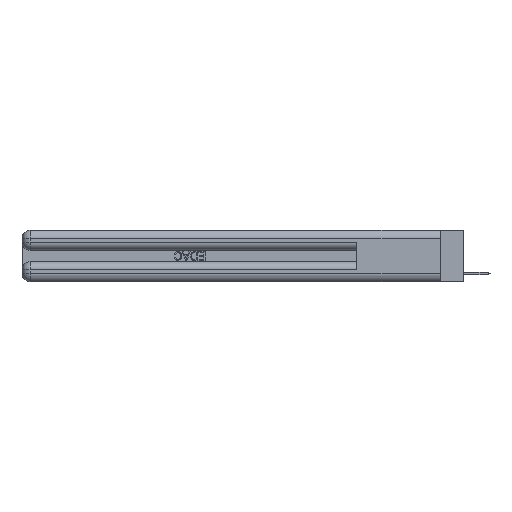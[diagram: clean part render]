
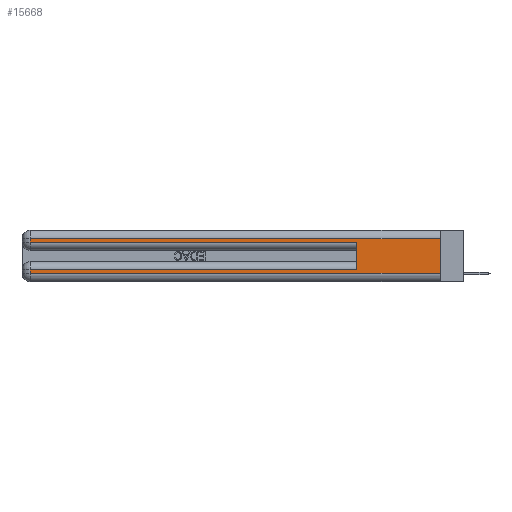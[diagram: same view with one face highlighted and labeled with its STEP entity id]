
A CAD part, left-side view. The second image highlights one B-rep face of the part: STEP entity #15668.
In plain terms, the highlighted planar face has unit normal (-1, 0, 0).
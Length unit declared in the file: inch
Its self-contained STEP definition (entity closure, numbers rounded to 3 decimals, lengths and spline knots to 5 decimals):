
#239 = VECTOR ( 'NONE', #15627, 39.37008 ) ;
#429 = CARTESIAN_POINT ( 'NONE',  ( 0., 0., 0.31 ) ) ;
#573 = EDGE_CURVE ( 'NONE', #22714, #7051, #14240, .T. ) ;
#1526 = ORIENTED_EDGE ( 'NONE', *, *, #16841, .T. ) ;
#1553 = VERTEX_POINT ( 'NONE', #7938 ) ;
#2909 = CARTESIAN_POINT ( 'NONE',  ( 0., 2.94, 0.31 ) ) ;
#2982 = CARTESIAN_POINT ( 'NONE',  ( 0., 0., 0.285 ) ) ;
#3354 = PLANE ( 'NONE',  #17115 ) ;
#3477 = ORIENTED_EDGE ( 'NONE', *, *, #8766, .T. ) ;
#3708 = ORIENTED_EDGE ( 'NONE', *, *, #11903, .T. ) ;
#3887 = EDGE_LOOP ( 'NONE', ( #17079, #9381, #19262, #3708, #11770, #1526, #8779, #3477 ) ) ;
#4520 = VECTOR ( 'NONE', #27031, 39.37008 ) ;
#4703 = CARTESIAN_POINT ( 'NONE',  ( 0., 2.94, 0.285 ) ) ;
#4941 = VERTEX_POINT ( 'NONE', #2909 ) ;
#5452 = CARTESIAN_POINT ( 'NONE',  ( 0., 0.6, 0.145 ) ) ;
#5494 = DIRECTION ( 'NONE',  ( 0., 0., -1. ) ) ;
#5507 = EDGE_CURVE ( 'NONE', #13946, #19288, #10993, .T. ) ;
#6389 = CARTESIAN_POINT ( 'NONE',  ( 0., 0.6, 0.085 ) ) ;
#7051 = VERTEX_POINT ( 'NONE', #27505 ) ;
#7171 = VECTOR ( 'NONE', #9244, 39.37008 ) ;
#7185 = CARTESIAN_POINT ( 'NONE',  ( 0., 2.94, 0.37 ) ) ;
#7938 = CARTESIAN_POINT ( 'NONE',  ( 0., 0.6, 0.285 ) ) ;
#8766 = EDGE_CURVE ( 'NONE', #19288, #7051, #10172, .T. ) ;
#8779 = ORIENTED_EDGE ( 'NONE', *, *, #5507, .T. ) ;
#8797 = LINE ( 'NONE', #5452, #7171 ) ;
#8917 = EDGE_CURVE ( 'NONE', #22714, #4941, #16277, .T. ) ;
#9050 = FACE_OUTER_BOUND ( 'NONE', #3887, .T. ) ;
#9244 = DIRECTION ( 'NONE',  ( 0., 0., 1. ) ) ;
#9381 = ORIENTED_EDGE ( 'NONE', *, *, #8917, .T. ) ;
#9525 = DIRECTION ( 'NONE',  ( 0., 1., 0. ) ) ;
#10096 = DIRECTION ( 'NONE',  ( 0., 0., -1. ) ) ;
#10172 = LINE ( 'NONE', #11922, #4520 ) ;
#10226 = VECTOR ( 'NONE', #11523, 39.37008 ) ;
#10326 = VECTOR ( 'NONE', #19704, 39.37008 ) ;
#10636 = CARTESIAN_POINT ( 'NONE',  ( 0., 0., 0.31 ) ) ;
#10993 = LINE ( 'NONE', #7185, #10326 ) ;
#11523 = DIRECTION ( 'NONE',  ( 0., -1., 0. ) ) ;
#11770 = ORIENTED_EDGE ( 'NONE', *, *, #24814, .F. ) ;
#11775 = CARTESIAN_POINT ( 'NONE',  ( 0., 2.94, 0.37 ) ) ;
#11903 = EDGE_CURVE ( 'NONE', #18441, #1553, #27255, .T. ) ;
#11922 = CARTESIAN_POINT ( 'NONE',  ( 0., 0., 0.06 ) ) ;
#12849 = CARTESIAN_POINT ( 'NONE',  ( 0., 2.94, 0.085 ) ) ;
#13946 = VERTEX_POINT ( 'NONE', #12849 ) ;
#14240 = LINE ( 'NONE', #21968, #239 ) ;
#14255 = CARTESIAN_POINT ( 'NONE',  ( 0., 2.94, 0.06 ) ) ;
#14999 = VECTOR ( 'NONE', #18984, 39.37008 ) ;
#15140 = LINE ( 'NONE', #11775, #25824 ) ;
#15627 = DIRECTION ( 'NONE',  ( 0., 0., -1. ) ) ;
#15668 = ADVANCED_FACE ( 'NONE', ( #9050 ), #3354, .F. ) ;
#16277 = LINE ( 'NONE', #10636, #26973 ) ;
#16841 = EDGE_CURVE ( 'NONE', #20194, #13946, #19969, .T. ) ;
#17079 = ORIENTED_EDGE ( 'NONE', *, *, #573, .F. ) ;
#17115 = AXIS2_PLACEMENT_3D ( 'NONE', #22604, #24765, #5494 ) ;
#18441 = VERTEX_POINT ( 'NONE', #4703 ) ;
#18984 = DIRECTION ( 'NONE',  ( 0., 1., 0. ) ) ;
#19262 = ORIENTED_EDGE ( 'NONE', *, *, #21083, .T. ) ;
#19288 = VERTEX_POINT ( 'NONE', #14255 ) ;
#19704 = DIRECTION ( 'NONE',  ( 0., 0., -1. ) ) ;
#19969 = LINE ( 'NONE', #25441, #14999 ) ;
#20194 = VERTEX_POINT ( 'NONE', #6389 ) ;
#21083 = EDGE_CURVE ( 'NONE', #4941, #18441, #15140, .T. ) ;
#21968 = CARTESIAN_POINT ( 'NONE',  ( 0., 0., 0.37 ) ) ;
#22604 = CARTESIAN_POINT ( 'NONE',  ( 0., 0., 0.37 ) ) ;
#22714 = VERTEX_POINT ( 'NONE', #429 ) ;
#24765 = DIRECTION ( 'NONE',  ( 1., 0., 0. ) ) ;
#24814 = EDGE_CURVE ( 'NONE', #20194, #1553, #8797, .T. ) ;
#25441 = CARTESIAN_POINT ( 'NONE',  ( 0., 0., 0.085 ) ) ;
#25824 = VECTOR ( 'NONE', #10096, 39.37008 ) ;
#26973 = VECTOR ( 'NONE', #9525, 39.37008 ) ;
#27031 = DIRECTION ( 'NONE',  ( 0., -1., 0. ) ) ;
#27255 = LINE ( 'NONE', #2982, #10226 ) ;
#27505 = CARTESIAN_POINT ( 'NONE',  ( 0., 0., 0.06 ) ) ;
